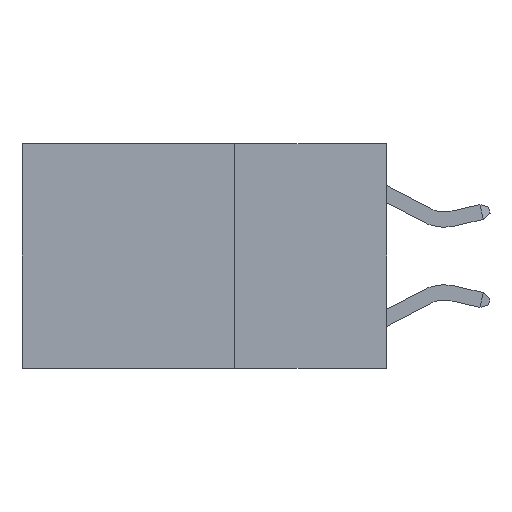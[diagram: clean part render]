
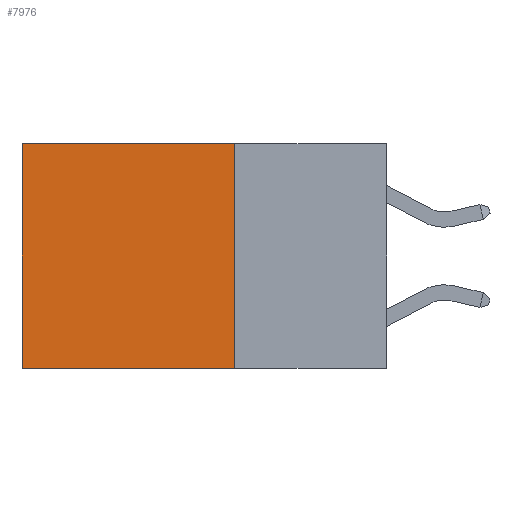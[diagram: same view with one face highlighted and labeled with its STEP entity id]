
A CAD part, left-side view. The second image highlights one B-rep face of the part: STEP entity #7976.
In plain terms, the highlighted planar face has unit normal (-1, 0, 0).
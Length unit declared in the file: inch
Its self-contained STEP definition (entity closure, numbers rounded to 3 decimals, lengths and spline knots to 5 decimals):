
#82 = CARTESIAN_POINT ( 'NONE',  ( 0.2625, 0.25, 0. ) ) ;
#451 = EDGE_CURVE ( 'NONE', #18237, #19452, #19233, .T. ) ;
#1666 = VECTOR ( 'NONE', #24953, 39.37008 ) ;
#1785 = VECTOR ( 'NONE', #4465, 39.37008 ) ;
#3273 = DIRECTION ( 'NONE',  ( 0., 0., -1. ) ) ;
#4103 = VERTEX_POINT ( 'NONE', #7039 ) ;
#4261 = ORIENTED_EDGE ( 'NONE', *, *, #5667, .T. ) ;
#4465 = DIRECTION ( 'NONE',  ( 0., 0., -1. ) ) ;
#5353 = FACE_OUTER_BOUND ( 'NONE', #25984, .T. ) ;
#5667 = EDGE_CURVE ( 'NONE', #18237, #8246, #20033, .T. ) ;
#7031 = VECTOR ( 'NONE', #20036, 39.37008 ) ;
#7039 = CARTESIAN_POINT ( 'NONE',  ( 0.2625, 0.6, -0.37 ) ) ;
#7182 = ORIENTED_EDGE ( 'NONE', *, *, #10070, .T. ) ;
#7471 = LINE ( 'NONE', #24204, #7031 ) ;
#7927 = EDGE_CURVE ( 'NONE', #19452, #4103, #7471, .T. ) ;
#7976 = ADVANCED_FACE ( 'NONE', ( #5353 ), #11258, .F. ) ;
#8246 = VERTEX_POINT ( 'NONE', #12640 ) ;
#8672 = VECTOR ( 'NONE', #9442, 39.37008 ) ;
#9442 = DIRECTION ( 'NONE',  ( 0., 1., 0. ) ) ;
#9446 = CARTESIAN_POINT ( 'NONE',  ( 0.2625, 0.25, 0. ) ) ;
#10070 = EDGE_CURVE ( 'NONE', #8246, #4103, #19430, .T. ) ;
#10294 = CARTESIAN_POINT ( 'NONE',  ( 0.2625, 0.25, 0. ) ) ;
#11258 = PLANE ( 'NONE',  #25769 ) ;
#12092 = ORIENTED_EDGE ( 'NONE', *, *, #7927, .F. ) ;
#12640 = CARTESIAN_POINT ( 'NONE',  ( 0.2625, 0.6, 0. ) ) ;
#12773 = ORIENTED_EDGE ( 'NONE', *, *, #451, .F. ) ;
#13908 = DIRECTION ( 'NONE',  ( 1., 0., 0. ) ) ;
#16198 = CARTESIAN_POINT ( 'NONE',  ( 0.2625, 0.25, -0.37 ) ) ;
#18237 = VERTEX_POINT ( 'NONE', #10294 ) ;
#19233 = LINE ( 'NONE', #82, #1666 ) ;
#19430 = LINE ( 'NONE', #25696, #1785 ) ;
#19452 = VERTEX_POINT ( 'NONE', #16198 ) ;
#20033 = LINE ( 'NONE', #24627, #8672 ) ;
#20036 = DIRECTION ( 'NONE',  ( 0., 1., 0. ) ) ;
#24204 = CARTESIAN_POINT ( 'NONE',  ( 0.2625, 0.25, -0.37 ) ) ;
#24627 = CARTESIAN_POINT ( 'NONE',  ( 0.2625, 0.25, 0. ) ) ;
#24953 = DIRECTION ( 'NONE',  ( 0., 0., -1. ) ) ;
#25696 = CARTESIAN_POINT ( 'NONE',  ( 0.2625, 0.6, 0. ) ) ;
#25769 = AXIS2_PLACEMENT_3D ( 'NONE', #9446, #13908, #3273 ) ;
#25984 = EDGE_LOOP ( 'NONE', ( #7182, #12092, #12773, #4261 ) ) ;
